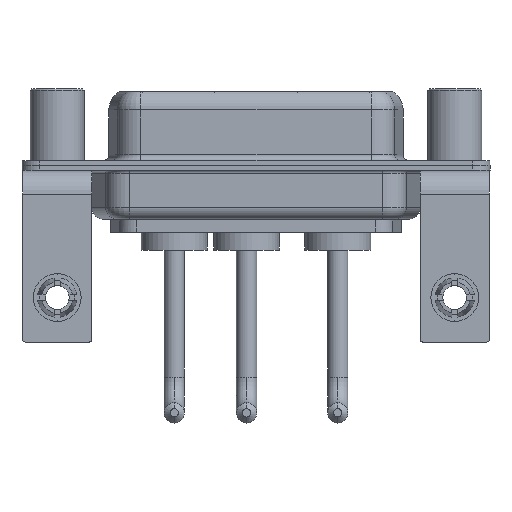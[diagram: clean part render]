
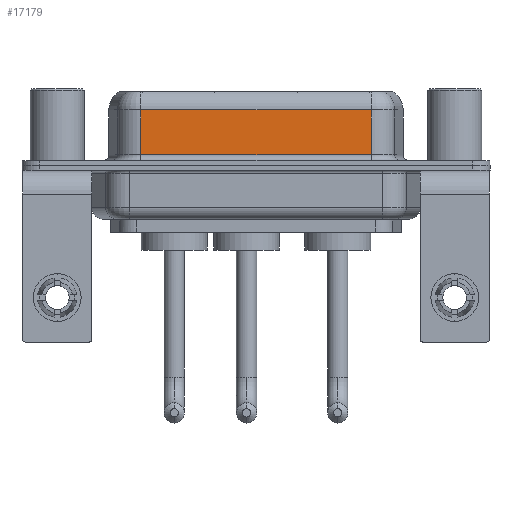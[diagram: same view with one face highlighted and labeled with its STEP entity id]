
A CAD part, front view. The second image highlights one B-rep face of the part: STEP entity #17179.
In plain terms, the highlighted planar face has unit normal (0, -1, 0).
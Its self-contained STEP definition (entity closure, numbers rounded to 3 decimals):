
#626 = CARTESIAN_POINT ( 'NONE',  ( 26.287, -3.95, 6.4 ) ) ;
#627 = EDGE_CURVE ( 'NONE', #4130, #7654, #12302, .T. ) ;
#712 = PLANE ( 'NONE',  #11887 ) ;
#1030 = CARTESIAN_POINT ( 'NONE',  ( 7.013, -3.95, 4.65 ) ) ;
#1375 = VECTOR ( 'NONE', #4421, 1000. ) ;
#1415 = VECTOR ( 'NONE', #6494, 1000. ) ;
#1445 = ORIENTED_EDGE ( 'NONE', *, *, #2230, .T. ) ;
#2071 = FACE_OUTER_BOUND ( 'NONE', #13742, .T. ) ;
#2230 = EDGE_CURVE ( 'NONE', #7654, #6250, #6022, .T. ) ;
#4038 = CARTESIAN_POINT ( 'NONE',  ( 26.287, -3.95, 4.65 ) ) ;
#4130 = VERTEX_POINT ( 'NONE', #17239 ) ;
#4421 = DIRECTION ( 'NONE',  ( 1., 0., 0. ) ) ;
#5886 = CARTESIAN_POINT ( 'NONE',  ( 26.287, -3.95, 0.9 ) ) ;
#6022 = LINE ( 'NONE', #11824, #13337 ) ;
#6165 = DIRECTION ( 'NONE',  ( 0., 0., 1. ) ) ;
#6250 = VERTEX_POINT ( 'NONE', #17064 ) ;
#6343 = DIRECTION ( 'NONE',  ( 0., 1., 0. ) ) ;
#6494 = DIRECTION ( 'NONE',  ( -1., 0., 0. ) ) ;
#6898 = ORIENTED_EDGE ( 'NONE', *, *, #627, .T. ) ;
#7477 = DIRECTION ( 'NONE',  ( 0., 0., -1. ) ) ;
#7654 = VERTEX_POINT ( 'NONE', #1030 ) ;
#7808 = CARTESIAN_POINT ( 'NONE',  ( 26.287, -3.95, 0.9 ) ) ;
#8123 = VERTEX_POINT ( 'NONE', #7808 ) ;
#8539 = EDGE_CURVE ( 'NONE', #6250, #8123, #16853, .T. ) ;
#9216 = CARTESIAN_POINT ( 'NONE',  ( 26.287, -3.95, 6.4 ) ) ;
#9486 = VECTOR ( 'NONE', #10945, 1000. ) ;
#10945 = DIRECTION ( 'NONE',  ( 0., 0., -1. ) ) ;
#11128 = ORIENTED_EDGE ( 'NONE', *, *, #15447, .F. ) ;
#11824 = CARTESIAN_POINT ( 'NONE',  ( 7.013, -3.95, 6.4 ) ) ;
#11887 = AXIS2_PLACEMENT_3D ( 'NONE', #626, #6343, #6165 ) ;
#12302 = LINE ( 'NONE', #4038, #1415 ) ;
#13337 = VECTOR ( 'NONE', #7477, 1000. ) ;
#13742 = EDGE_LOOP ( 'NONE', ( #11128, #6898, #1445, #14157 ) ) ;
#14157 = ORIENTED_EDGE ( 'NONE', *, *, #8539, .T. ) ;
#15447 = EDGE_CURVE ( 'NONE', #4130, #8123, #17739, .T. ) ;
#16853 = LINE ( 'NONE', #5886, #1375 ) ;
#17064 = CARTESIAN_POINT ( 'NONE',  ( 7.013, -3.95, 0.9 ) ) ;
#17179 = ADVANCED_FACE ( 'NONE', ( #2071 ), #712, .F. ) ;
#17239 = CARTESIAN_POINT ( 'NONE',  ( 26.287, -3.95, 4.65 ) ) ;
#17739 = LINE ( 'NONE', #9216, #9486 ) ;
